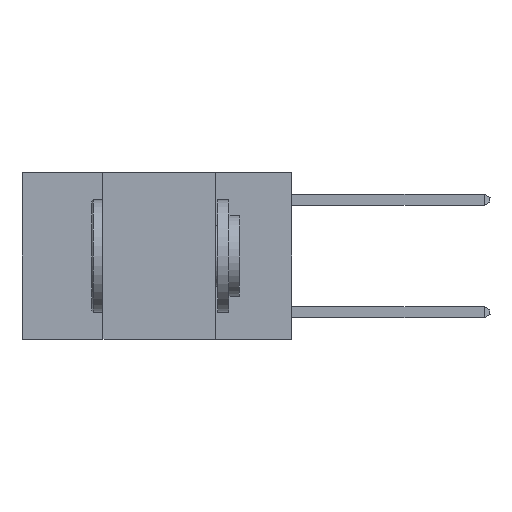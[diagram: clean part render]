
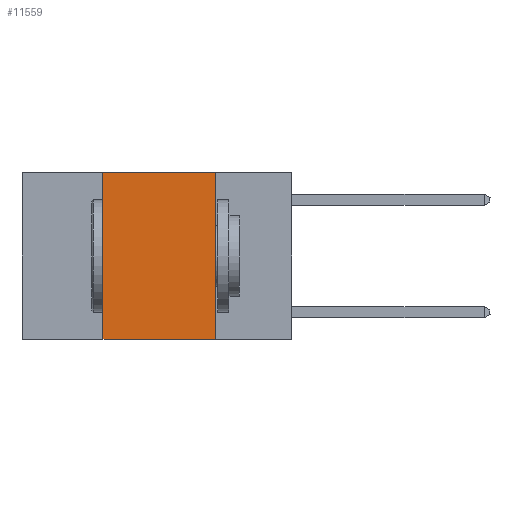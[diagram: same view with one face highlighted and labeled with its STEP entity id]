
A CAD part, left-side view. The second image highlights one B-rep face of the part: STEP entity #11559.
In plain terms, the highlighted planar face has unit normal (-1, 0, 0).
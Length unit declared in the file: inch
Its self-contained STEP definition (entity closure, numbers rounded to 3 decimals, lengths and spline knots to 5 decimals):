
#1468 = CARTESIAN_POINT ( 'NONE',  ( 0., 0.42, -0.37 ) ) ;
#1531 = EDGE_CURVE ( 'NONE', #5053, #10773, #14134, .T. ) ;
#1794 = DIRECTION ( 'NONE',  ( 0., -1., 0. ) ) ;
#1872 = EDGE_CURVE ( 'NONE', #2752, #5053, #14328, .T. ) ;
#2027 = PLANE ( 'NONE',  #15463 ) ;
#2146 = CARTESIAN_POINT ( 'NONE',  ( 0., 0.6, 0. ) ) ;
#2752 = VERTEX_POINT ( 'NONE', #16268 ) ;
#3511 = VECTOR ( 'NONE', #21235, 39.37008 ) ;
#3536 = FACE_OUTER_BOUND ( 'NONE', #19522, .T. ) ;
#3779 = LINE ( 'NONE', #14599, #5827 ) ;
#4543 = LINE ( 'NONE', #16654, #16441 ) ;
#5053 = VERTEX_POINT ( 'NONE', #13280 ) ;
#5827 = VECTOR ( 'NONE', #11119, 39.37008 ) ;
#6176 = VERTEX_POINT ( 'NONE', #1468 ) ;
#7298 = EDGE_CURVE ( 'NONE', #6176, #10773, #3779, .T. ) ;
#8376 = ORIENTED_EDGE ( 'NONE', *, *, #7298, .T. ) ;
#10773 = VERTEX_POINT ( 'NONE', #13155 ) ;
#10981 = DIRECTION ( 'NONE',  ( 0., 0., -1. ) ) ;
#11119 = DIRECTION ( 'NONE',  ( 0., -1., 0. ) ) ;
#11559 = ADVANCED_FACE ( 'NONE', ( #3536 ), #2027, .F. ) ;
#13155 = CARTESIAN_POINT ( 'NONE',  ( 0., 0.17, -0.37 ) ) ;
#13280 = CARTESIAN_POINT ( 'NONE',  ( 0., 0.17, 0. ) ) ;
#13555 = ORIENTED_EDGE ( 'NONE', *, *, #1531, .F. ) ;
#13589 = EDGE_CURVE ( 'NONE', #6176, #2752, #4543, .T. ) ;
#14134 = LINE ( 'NONE', #16115, #3511 ) ;
#14328 = LINE ( 'NONE', #21095, #14670 ) ;
#14475 = DIRECTION ( 'NONE',  ( 1., 0., 0. ) ) ;
#14599 = CARTESIAN_POINT ( 'NONE',  ( 0., 0.6, -0.37 ) ) ;
#14670 = VECTOR ( 'NONE', #1794, 39.37008 ) ;
#15463 = AXIS2_PLACEMENT_3D ( 'NONE', #2146, #14475, #10981 ) ;
#16115 = CARTESIAN_POINT ( 'NONE',  ( 0., 0.17, 0. ) ) ;
#16268 = CARTESIAN_POINT ( 'NONE',  ( 0., 0.42, 0. ) ) ;
#16441 = VECTOR ( 'NONE', #18627, 39.37008 ) ;
#16654 = CARTESIAN_POINT ( 'NONE',  ( 0., 0.42, 0. ) ) ;
#18627 = DIRECTION ( 'NONE',  ( 0., 0., 1. ) ) ;
#19514 = ORIENTED_EDGE ( 'NONE', *, *, #1872, .F. ) ;
#19522 = EDGE_LOOP ( 'NONE', ( #13555, #19514, #20995, #8376 ) ) ;
#20995 = ORIENTED_EDGE ( 'NONE', *, *, #13589, .F. ) ;
#21095 = CARTESIAN_POINT ( 'NONE',  ( 0., 0.6, 0. ) ) ;
#21235 = DIRECTION ( 'NONE',  ( 0., 0., -1. ) ) ;
